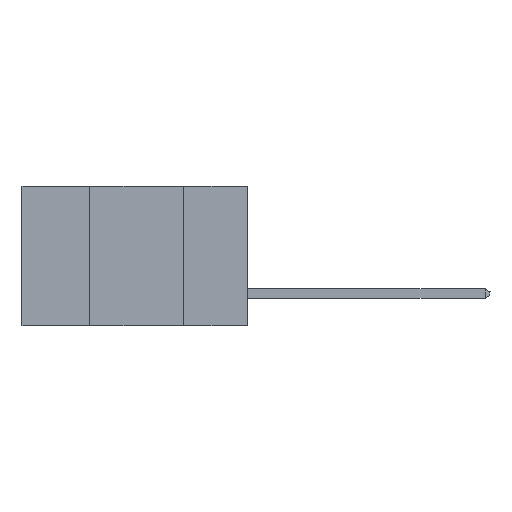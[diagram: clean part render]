
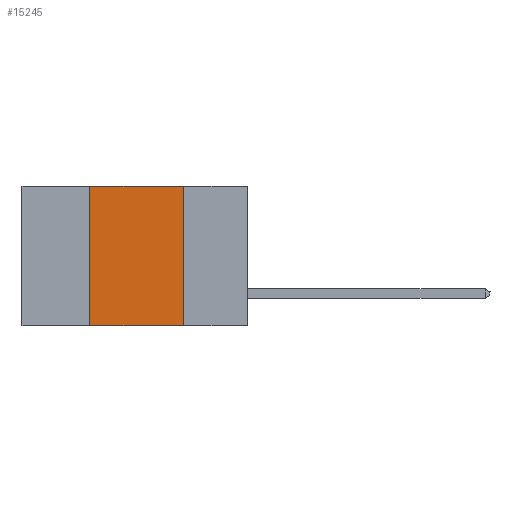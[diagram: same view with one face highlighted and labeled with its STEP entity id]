
A CAD part, left-side view. The second image highlights one B-rep face of the part: STEP entity #15245.
In plain terms, the highlighted planar face has unit normal (-1, 0, 0).
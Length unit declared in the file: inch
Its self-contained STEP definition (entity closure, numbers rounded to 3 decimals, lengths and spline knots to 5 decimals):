
#77 = VECTOR ( 'NONE', #18317, 39.37008 ) ;
#110 = LINE ( 'NONE', #6599, #77 ) ;
#310 = LINE ( 'NONE', #15018, #10411 ) ;
#449 = VERTEX_POINT ( 'NONE', #8459 ) ;
#873 = EDGE_CURVE ( 'NONE', #5228, #20428, #110, .T. ) ;
#1310 = ORIENTED_EDGE ( 'NONE', *, *, #2483, .T. ) ;
#2015 = DIRECTION ( 'NONE',  ( 0., -1., 0. ) ) ;
#2075 = AXIS2_PLACEMENT_3D ( 'NONE', #4722, #3118, #16114 ) ;
#2483 = EDGE_CURVE ( 'NONE', #449, #7849, #310, .T. ) ;
#2619 = CARTESIAN_POINT ( 'NONE',  ( 0., 0.42, -0.37 ) ) ;
#3118 = DIRECTION ( 'NONE',  ( 1., 0., 0. ) ) ;
#3424 = CARTESIAN_POINT ( 'NONE',  ( 0., 0.17, 0. ) ) ;
#3552 = ORIENTED_EDGE ( 'NONE', *, *, #9834, .F. ) ;
#4328 = ORIENTED_EDGE ( 'NONE', *, *, #873, .F. ) ;
#4722 = CARTESIAN_POINT ( 'NONE',  ( 0., 0.6, 0. ) ) ;
#4933 = EDGE_LOOP ( 'NONE', ( #13750, #4328, #3552, #1310 ) ) ;
#5228 = VERTEX_POINT ( 'NONE', #6832 ) ;
#5389 = CARTESIAN_POINT ( 'NONE',  ( 0., 0.17, -0.37 ) ) ;
#6312 = FACE_OUTER_BOUND ( 'NONE', #4933, .T. ) ;
#6599 = CARTESIAN_POINT ( 'NONE',  ( 0., 0.6, 0. ) ) ;
#6832 = CARTESIAN_POINT ( 'NONE',  ( 0., 0.42, 0. ) ) ;
#7849 = VERTEX_POINT ( 'NONE', #15469 ) ;
#8459 = CARTESIAN_POINT ( 'NONE',  ( 0., 0.42, -0.37 ) ) ;
#9834 = EDGE_CURVE ( 'NONE', #449, #5228, #20380, .T. ) ;
#10411 = VECTOR ( 'NONE', #2015, 39.37008 ) ;
#11971 = VECTOR ( 'NONE', #20281, 39.37008 ) ;
#12825 = PLANE ( 'NONE',  #2075 ) ;
#13462 = VECTOR ( 'NONE', #20265, 39.37008 ) ;
#13750 = ORIENTED_EDGE ( 'NONE', *, *, #17393, .F. ) ;
#15018 = CARTESIAN_POINT ( 'NONE',  ( 0., 0.6, -0.37 ) ) ;
#15245 = ADVANCED_FACE ( 'NONE', ( #6312 ), #12825, .F. ) ;
#15469 = CARTESIAN_POINT ( 'NONE',  ( 0., 0.17, -0.37 ) ) ;
#16114 = DIRECTION ( 'NONE',  ( 0., 0., -1. ) ) ;
#17393 = EDGE_CURVE ( 'NONE', #20428, #7849, #19964, .T. ) ;
#18317 = DIRECTION ( 'NONE',  ( 0., -1., 0. ) ) ;
#19964 = LINE ( 'NONE', #5389, #13462 ) ;
#20265 = DIRECTION ( 'NONE',  ( 0., 0., -1. ) ) ;
#20281 = DIRECTION ( 'NONE',  ( 0., 0., 1. ) ) ;
#20380 = LINE ( 'NONE', #2619, #11971 ) ;
#20428 = VERTEX_POINT ( 'NONE', #3424 ) ;
